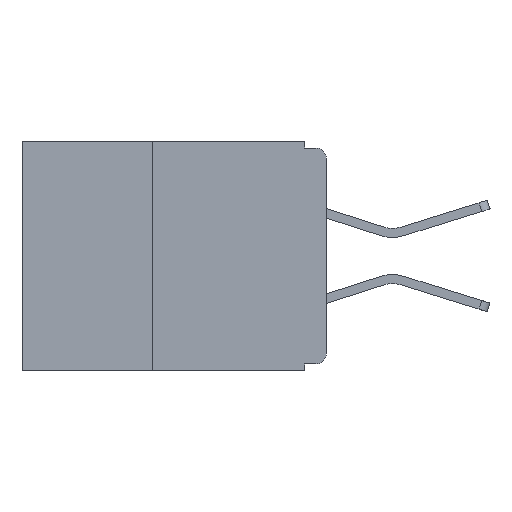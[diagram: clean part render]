
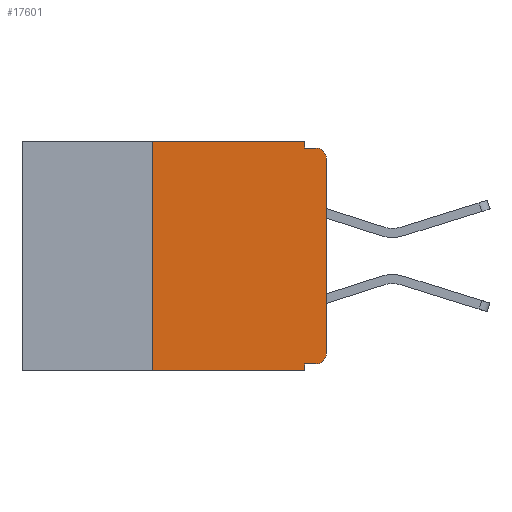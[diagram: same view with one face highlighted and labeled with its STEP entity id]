
A CAD part, left-side view. The second image highlights one B-rep face of the part: STEP entity #17601.
In plain terms, the highlighted planar face has unit normal (-1, 0, 0).
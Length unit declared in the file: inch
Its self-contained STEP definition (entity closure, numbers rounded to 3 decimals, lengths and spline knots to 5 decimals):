
#74 = CARTESIAN_POINT ( 'NONE',  ( 0., 0.031, 0. ) ) ;
#342 = AXIS2_PLACEMENT_3D ( 'NONE', #4176, #6315, #21113 ) ;
#382 = LINE ( 'NONE', #8313, #22356 ) ;
#683 = AXIS2_PLACEMENT_3D ( 'NONE', #15804, #15755, #15748 ) ;
#952 = CARTESIAN_POINT ( 'NONE',  ( 0., 0.015, -0.01 ) ) ;
#1037 = EDGE_CURVE ( 'NONE', #15501, #18496, #6855, .T. ) ;
#1771 = CARTESIAN_POINT ( 'NONE',  ( 0., 0.031, -0.33 ) ) ;
#1775 = ORIENTED_EDGE ( 'NONE', *, *, #10260, .T. ) ;
#1910 = DIRECTION ( 'NONE',  ( 0., 0., 1. ) ) ;
#2144 = ORIENTED_EDGE ( 'NONE', *, *, #5965, .T. ) ;
#2355 = VERTEX_POINT ( 'NONE', #8646 ) ;
#2371 = LINE ( 'NONE', #26676, #7425 ) ;
#2516 = VERTEX_POINT ( 'NONE', #21178 ) ;
#2557 = VECTOR ( 'NONE', #10432, 39.37008 ) ;
#2682 = DIRECTION ( 'NONE',  ( 0., -1., 0. ) ) ;
#3408 = VECTOR ( 'NONE', #25063, 39.37008 ) ;
#3882 = EDGE_CURVE ( 'NONE', #24786, #8510, #2371, .T. ) ;
#4176 = CARTESIAN_POINT ( 'NONE',  ( 0., 0.437, 0. ) ) ;
#4500 = LINE ( 'NONE', #74, #5170 ) ;
#4742 = VERTEX_POINT ( 'NONE', #13792 ) ;
#5093 = CARTESIAN_POINT ( 'NONE',  ( 0., 0., 0. ) ) ;
#5137 = DIRECTION ( 'NONE',  ( 0., 0., 1. ) ) ;
#5160 = VERTEX_POINT ( 'NONE', #7091 ) ;
#5170 = VECTOR ( 'NONE', #15151, 39.37008 ) ;
#5965 = EDGE_CURVE ( 'NONE', #4742, #15501, #17994, .T. ) ;
#6246 = AXIS2_PLACEMENT_3D ( 'NONE', #6370, #21162, #8511 ) ;
#6315 = DIRECTION ( 'NONE',  ( 1., 0., 0. ) ) ;
#6370 = CARTESIAN_POINT ( 'NONE',  ( 0., 0.015, -0.025 ) ) ;
#6537 = ORIENTED_EDGE ( 'NONE', *, *, #17552, .F. ) ;
#6855 = LINE ( 'NONE', #5093, #23604 ) ;
#7091 = CARTESIAN_POINT ( 'NONE',  ( 0., 0.031, -0.01 ) ) ;
#7350 = CARTESIAN_POINT ( 'NONE',  ( 0., 0., -0.305 ) ) ;
#7425 = VECTOR ( 'NONE', #26823, 39.37008 ) ;
#8257 = LINE ( 'NONE', #1771, #2557 ) ;
#8313 = CARTESIAN_POINT ( 'NONE',  ( 0., 0.25, -0.33 ) ) ;
#8510 = VERTEX_POINT ( 'NONE', #19534 ) ;
#8511 = DIRECTION ( 'NONE',  ( 0., 0., -1. ) ) ;
#8646 = CARTESIAN_POINT ( 'NONE',  ( 0., 0.031, -0.33 ) ) ;
#8848 = ORIENTED_EDGE ( 'NONE', *, *, #21695, .F. ) ;
#9101 = LINE ( 'NONE', #20977, #3408 ) ;
#9366 = CARTESIAN_POINT ( 'NONE',  ( 0., 0.25, 0. ) ) ;
#10198 = ORIENTED_EDGE ( 'NONE', *, *, #3882, .F. ) ;
#10260 = EDGE_CURVE ( 'NONE', #18496, #20061, #20876, .T. ) ;
#10432 = DIRECTION ( 'NONE',  ( 0., 0., -1. ) ) ;
#13792 = CARTESIAN_POINT ( 'NONE',  ( 0., 0.015, -0.32 ) ) ;
#13858 = ORIENTED_EDGE ( 'NONE', *, *, #20167, .F. ) ;
#14546 = EDGE_CURVE ( 'NONE', #4742, #2516, #9101, .T. ) ;
#15151 = DIRECTION ( 'NONE',  ( 0., 0., -1. ) ) ;
#15501 = VERTEX_POINT ( 'NONE', #7350 ) ;
#15748 = DIRECTION ( 'NONE',  ( 0., 0., -1. ) ) ;
#15755 = DIRECTION ( 'NONE',  ( -1., 0., 0. ) ) ;
#15804 = CARTESIAN_POINT ( 'NONE',  ( 0., 0.015, -0.305 ) ) ;
#15899 = VERTEX_POINT ( 'NONE', #19651 ) ;
#16097 = CARTESIAN_POINT ( 'NONE',  ( 0., 0., -0.025 ) ) ;
#16942 = PLANE ( 'NONE',  #342 ) ;
#17506 = ORIENTED_EDGE ( 'NONE', *, *, #1037, .T. ) ;
#17552 = EDGE_CURVE ( 'NONE', #2516, #2355, #8257, .T. ) ;
#17601 = ADVANCED_FACE ( 'NONE', ( #18241 ), #16942, .F. ) ;
#17914 = EDGE_LOOP ( 'NONE', ( #17506, #1775, #13858, #8848, #10198, #26746, #22670, #6537, #23316, #2144 ) ) ;
#17994 = CIRCLE ( 'NONE', #683, 0.015 ) ;
#18241 = FACE_OUTER_BOUND ( 'NONE', #17914, .T. ) ;
#18496 = VERTEX_POINT ( 'NONE', #16097 ) ;
#18529 = VECTOR ( 'NONE', #2682, 39.37008 ) ;
#18946 = EDGE_CURVE ( 'NONE', #15899, #2355, #23973, .T. ) ;
#19107 = VECTOR ( 'NONE', #24524, 39.37008 ) ;
#19534 = CARTESIAN_POINT ( 'NONE',  ( 0., 0.031, 0. ) ) ;
#19651 = CARTESIAN_POINT ( 'NONE',  ( 0., 0.25, -0.33 ) ) ;
#19752 = LINE ( 'NONE', #22492, #19107 ) ;
#20061 = VERTEX_POINT ( 'NONE', #952 ) ;
#20167 = EDGE_CURVE ( 'NONE', #5160, #20061, #19752, .T. ) ;
#20322 = EDGE_CURVE ( 'NONE', #15899, #24786, #382, .T. ) ;
#20876 = CIRCLE ( 'NONE', #6246, 0.015 ) ;
#20977 = CARTESIAN_POINT ( 'NONE',  ( 0., 0., -0.32 ) ) ;
#21113 = DIRECTION ( 'NONE',  ( 0., 0., -1. ) ) ;
#21162 = DIRECTION ( 'NONE',  ( -1., 0., 0. ) ) ;
#21178 = CARTESIAN_POINT ( 'NONE',  ( 0., 0.031, -0.32 ) ) ;
#21659 = CARTESIAN_POINT ( 'NONE',  ( 0., 0.437, -0.33 ) ) ;
#21695 = EDGE_CURVE ( 'NONE', #8510, #5160, #4500, .T. ) ;
#22356 = VECTOR ( 'NONE', #1910, 39.37008 ) ;
#22492 = CARTESIAN_POINT ( 'NONE',  ( 0., 0., -0.01 ) ) ;
#22670 = ORIENTED_EDGE ( 'NONE', *, *, #18946, .T. ) ;
#23316 = ORIENTED_EDGE ( 'NONE', *, *, #14546, .F. ) ;
#23604 = VECTOR ( 'NONE', #5137, 39.37008 ) ;
#23973 = LINE ( 'NONE', #21659, #18529 ) ;
#24524 = DIRECTION ( 'NONE',  ( 0., -1., 0. ) ) ;
#24786 = VERTEX_POINT ( 'NONE', #9366 ) ;
#25063 = DIRECTION ( 'NONE',  ( 0., 1., 0. ) ) ;
#26676 = CARTESIAN_POINT ( 'NONE',  ( 0., 0.437, 0. ) ) ;
#26746 = ORIENTED_EDGE ( 'NONE', *, *, #20322, .F. ) ;
#26823 = DIRECTION ( 'NONE',  ( 0., -1., 0. ) ) ;
